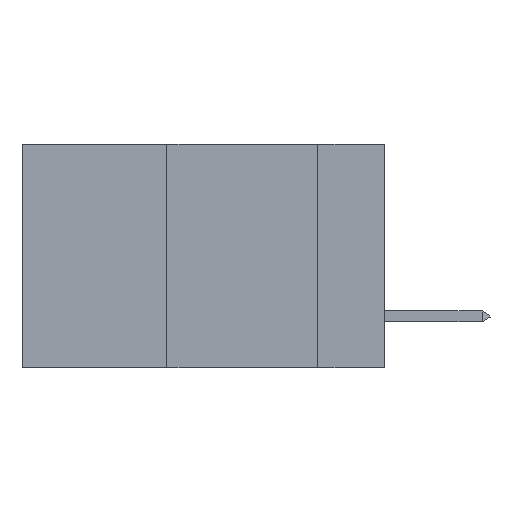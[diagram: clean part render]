
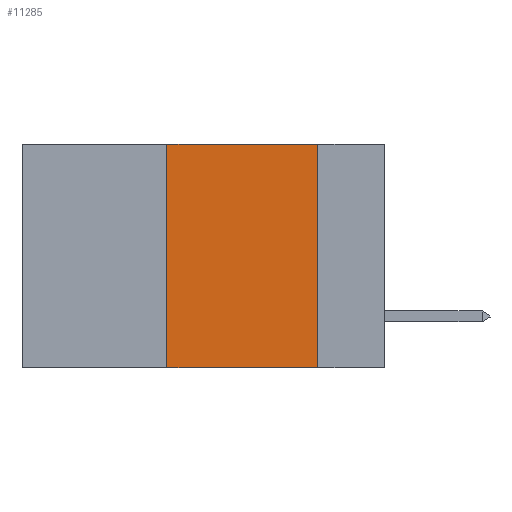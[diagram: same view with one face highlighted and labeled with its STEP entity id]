
A CAD part, left-side view. The second image highlights one B-rep face of the part: STEP entity #11285.
In plain terms, the highlighted planar face has unit normal (-1, 0, 0).
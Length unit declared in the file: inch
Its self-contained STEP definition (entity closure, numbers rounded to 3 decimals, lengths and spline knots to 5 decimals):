
#152 = ORIENTED_EDGE ( 'NONE', *, *, #5718, .T. ) ;
#265 = ORIENTED_EDGE ( 'NONE', *, *, #15554, .F. ) ;
#285 = DIRECTION ( 'NONE',  ( 0., 0., -1. ) ) ;
#944 = EDGE_CURVE ( 'NONE', #2227, #17534, #9588, .T. ) ;
#1096 = FACE_OUTER_BOUND ( 'NONE', #20184, .T. ) ;
#1478 = CARTESIAN_POINT ( 'NONE',  ( 0., 0.36, -0.37 ) ) ;
#1693 = CARTESIAN_POINT ( 'NONE',  ( 0., 0.11, -0.37 ) ) ;
#1798 = DIRECTION ( 'NONE',  ( 0., -1., 0. ) ) ;
#2227 = VERTEX_POINT ( 'NONE', #12990 ) ;
#2498 = PLANE ( 'NONE',  #5614 ) ;
#3424 = VECTOR ( 'NONE', #1798, 39.37008 ) ;
#4185 = DIRECTION ( 'NONE',  ( 1., 0., 0. ) ) ;
#4856 = VECTOR ( 'NONE', #8253, 39.37008 ) ;
#5431 = CARTESIAN_POINT ( 'NONE',  ( 0., 0.6, -0.37 ) ) ;
#5614 = AXIS2_PLACEMENT_3D ( 'NONE', #21299, #4185, #11214 ) ;
#5718 = EDGE_CURVE ( 'NONE', #15881, #20689, #8028, .T. ) ;
#6600 = VECTOR ( 'NONE', #285, 39.37008 ) ;
#8028 = LINE ( 'NONE', #5431, #19190 ) ;
#8253 = DIRECTION ( 'NONE',  ( 0., 0., 1. ) ) ;
#9588 = LINE ( 'NONE', #15302, #3424 ) ;
#9891 = EDGE_CURVE ( 'NONE', #15881, #2227, #13127, .T. ) ;
#10889 = CARTESIAN_POINT ( 'NONE',  ( 0., 0.11, 0. ) ) ;
#11214 = DIRECTION ( 'NONE',  ( 0., 0., -1. ) ) ;
#11285 = ADVANCED_FACE ( 'NONE', ( #1096 ), #2498, .F. ) ;
#11933 = ORIENTED_EDGE ( 'NONE', *, *, #944, .F. ) ;
#12990 = CARTESIAN_POINT ( 'NONE',  ( 0., 0.36, 0. ) ) ;
#13127 = LINE ( 'NONE', #13330, #4856 ) ;
#13330 = CARTESIAN_POINT ( 'NONE',  ( 0., 0.36, 0. ) ) ;
#15302 = CARTESIAN_POINT ( 'NONE',  ( 0., 0.6, 0. ) ) ;
#15554 = EDGE_CURVE ( 'NONE', #17534, #20689, #15983, .T. ) ;
#15744 = DIRECTION ( 'NONE',  ( 0., -1., 0. ) ) ;
#15881 = VERTEX_POINT ( 'NONE', #1478 ) ;
#15983 = LINE ( 'NONE', #10889, #6600 ) ;
#17534 = VERTEX_POINT ( 'NONE', #18601 ) ;
#18601 = CARTESIAN_POINT ( 'NONE',  ( 0., 0.11, 0. ) ) ;
#19190 = VECTOR ( 'NONE', #15744, 39.37008 ) ;
#20184 = EDGE_LOOP ( 'NONE', ( #265, #11933, #20741, #152 ) ) ;
#20689 = VERTEX_POINT ( 'NONE', #1693 ) ;
#20741 = ORIENTED_EDGE ( 'NONE', *, *, #9891, .F. ) ;
#21299 = CARTESIAN_POINT ( 'NONE',  ( 0., 0.6, 0. ) ) ;
